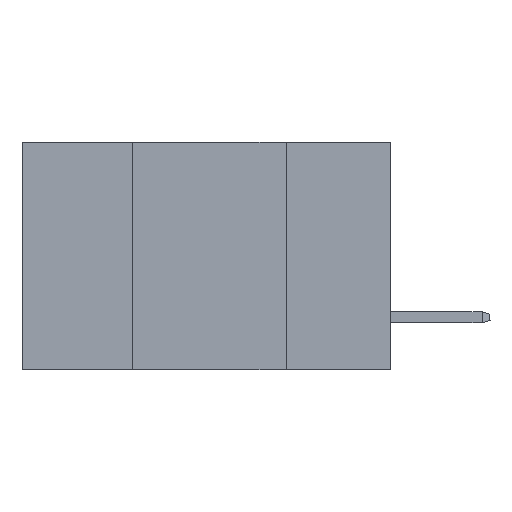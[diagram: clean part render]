
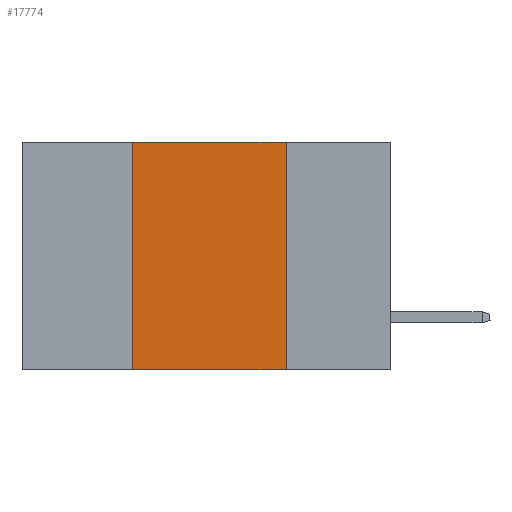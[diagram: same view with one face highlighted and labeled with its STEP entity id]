
A CAD part, left-side view. The second image highlights one B-rep face of the part: STEP entity #17774.
In plain terms, the highlighted planar face has unit normal (-1, 0, 0).
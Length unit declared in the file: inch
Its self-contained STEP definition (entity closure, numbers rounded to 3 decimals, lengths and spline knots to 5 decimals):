
#1 = VECTOR ( 'NONE', #12369, 39.37008 ) ;
#92 = EDGE_CURVE ( 'NONE', #11331, #25379, #19409, .T. ) ;
#3180 = CARTESIAN_POINT ( 'NONE',  ( 0., 0.42, 0. ) ) ;
#5371 = CARTESIAN_POINT ( 'NONE',  ( 0., 0.6, 0. ) ) ;
#5766 = CARTESIAN_POINT ( 'NONE',  ( 0., 0.6, -0.37 ) ) ;
#5799 = CARTESIAN_POINT ( 'NONE',  ( 0., 0.17, 0. ) ) ;
#5827 = VERTEX_POINT ( 'NONE', #14701 ) ;
#6201 = CARTESIAN_POINT ( 'NONE',  ( 0., 0.6, 0. ) ) ;
#8256 = ORIENTED_EDGE ( 'NONE', *, *, #24552, .F. ) ;
#10372 = VERTEX_POINT ( 'NONE', #12025 ) ;
#11331 = VERTEX_POINT ( 'NONE', #12051 ) ;
#11632 = DIRECTION ( 'NONE',  ( 0., 0., -1. ) ) ;
#11665 = DIRECTION ( 'NONE',  ( 0., 0., 1. ) ) ;
#12025 = CARTESIAN_POINT ( 'NONE',  ( 0., 0.42, -0.37 ) ) ;
#12051 = CARTESIAN_POINT ( 'NONE',  ( 0., 0.42, 0. ) ) ;
#12159 = EDGE_LOOP ( 'NONE', ( #8256, #21668, #32826, #24352 ) ) ;
#12369 = DIRECTION ( 'NONE',  ( 0., -1., 0. ) ) ;
#12942 = VECTOR ( 'NONE', #24670, 39.37008 ) ;
#13180 = DIRECTION ( 'NONE',  ( 0., 0., -1. ) ) ;
#14701 = CARTESIAN_POINT ( 'NONE',  ( 0., 0.17, -0.37 ) ) ;
#16142 = PLANE ( 'NONE',  #17272 ) ;
#16145 = VECTOR ( 'NONE', #11632, 39.37008 ) ;
#16551 = CARTESIAN_POINT ( 'NONE',  ( 0., 0.17, 0. ) ) ;
#17272 = AXIS2_PLACEMENT_3D ( 'NONE', #5371, #34835, #13180 ) ;
#17774 = ADVANCED_FACE ( 'NONE', ( #28176 ), #16142, .F. ) ;
#19409 = LINE ( 'NONE', #6201, #1 ) ;
#20143 = LINE ( 'NONE', #5766, #12942 ) ;
#21668 = ORIENTED_EDGE ( 'NONE', *, *, #92, .F. ) ;
#24352 = ORIENTED_EDGE ( 'NONE', *, *, #29102, .T. ) ;
#24552 = EDGE_CURVE ( 'NONE', #25379, #5827, #31732, .T. ) ;
#24670 = DIRECTION ( 'NONE',  ( 0., -1., 0. ) ) ;
#25379 = VERTEX_POINT ( 'NONE', #5799 ) ;
#28176 = FACE_OUTER_BOUND ( 'NONE', #12159, .T. ) ;
#29102 = EDGE_CURVE ( 'NONE', #10372, #5827, #20143, .T. ) ;
#31732 = LINE ( 'NONE', #16551, #16145 ) ;
#31741 = LINE ( 'NONE', #3180, #34652 ) ;
#32826 = ORIENTED_EDGE ( 'NONE', *, *, #33799, .F. ) ;
#33799 = EDGE_CURVE ( 'NONE', #10372, #11331, #31741, .T. ) ;
#34652 = VECTOR ( 'NONE', #11665, 39.37008 ) ;
#34835 = DIRECTION ( 'NONE',  ( 1., 0., 0. ) ) ;
